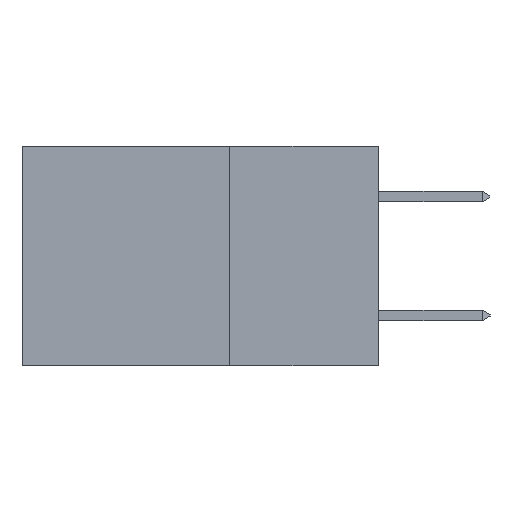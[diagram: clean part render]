
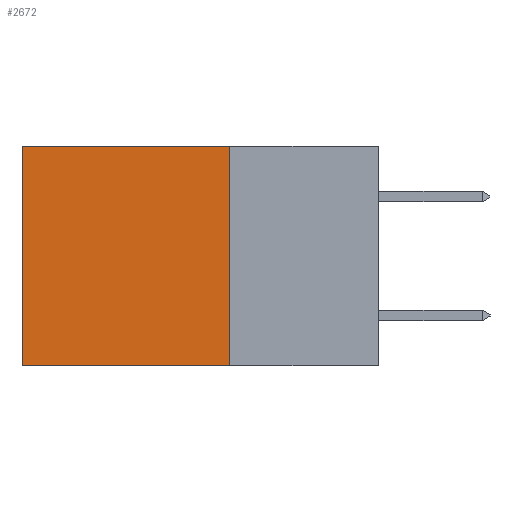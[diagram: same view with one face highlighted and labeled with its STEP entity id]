
A CAD part, left-side view. The second image highlights one B-rep face of the part: STEP entity #2672.
In plain terms, the highlighted planar face has unit normal (-1, 0, 0).
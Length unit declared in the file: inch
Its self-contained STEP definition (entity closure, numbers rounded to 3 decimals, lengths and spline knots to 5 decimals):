
#206 = AXIS2_PLACEMENT_3D ( 'NONE', #6173, #8094, #4147 ) ;
#280 = CARTESIAN_POINT ( 'NONE',  ( 0.2615, 0.25, -0.37 ) ) ;
#621 = EDGE_CURVE ( 'NONE', #991, #4308, #4250, .T. ) ;
#991 = VERTEX_POINT ( 'NONE', #280 ) ;
#1188 = DIRECTION ( 'NONE',  ( 0., 0., -1. ) ) ;
#1321 = CARTESIAN_POINT ( 'NONE',  ( 0.2615, 0.6, -0.37 ) ) ;
#1491 = EDGE_CURVE ( 'NONE', #3774, #991, #6326, .T. ) ;
#1506 = CARTESIAN_POINT ( 'NONE',  ( 0.2615, 0.25, -0.37 ) ) ;
#1646 = LINE ( 'NONE', #1321, #3534 ) ;
#2672 = ADVANCED_FACE ( 'NONE', ( #2991 ), #7448, .F. ) ;
#2991 = FACE_OUTER_BOUND ( 'NONE', #8503, .T. ) ;
#3029 = ORIENTED_EDGE ( 'NONE', *, *, #5022, .T. ) ;
#3534 = VECTOR ( 'NONE', #3707, 39.37008 ) ;
#3707 = DIRECTION ( 'NONE',  ( 0., 0., -1. ) ) ;
#3774 = VERTEX_POINT ( 'NONE', #5849 ) ;
#4147 = DIRECTION ( 'NONE',  ( 0., 0., -1. ) ) ;
#4250 = LINE ( 'NONE', #8840, #7572 ) ;
#4308 = VERTEX_POINT ( 'NONE', #5204 ) ;
#4875 = DIRECTION ( 'NONE',  ( 0., 1., 0. ) ) ;
#5022 = EDGE_CURVE ( 'NONE', #3774, #5112, #8647, .T. ) ;
#5112 = VERTEX_POINT ( 'NONE', #6967 ) ;
#5204 = CARTESIAN_POINT ( 'NONE',  ( 0.2615, 0.6, -0.37 ) ) ;
#5849 = CARTESIAN_POINT ( 'NONE',  ( 0.2615, 0.25, 0. ) ) ;
#6125 = VECTOR ( 'NONE', #1188, 39.37008 ) ;
#6173 = CARTESIAN_POINT ( 'NONE',  ( 0.2615, 0.25, -0.37 ) ) ;
#6222 = ORIENTED_EDGE ( 'NONE', *, *, #6470, .T. ) ;
#6326 = LINE ( 'NONE', #1506, #6125 ) ;
#6470 = EDGE_CURVE ( 'NONE', #5112, #4308, #1646, .T. ) ;
#6821 = ORIENTED_EDGE ( 'NONE', *, *, #621, .F. ) ;
#6967 = CARTESIAN_POINT ( 'NONE',  ( 0.2615, 0.6, 0. ) ) ;
#7337 = DIRECTION ( 'NONE',  ( 0., 1., 0. ) ) ;
#7448 = PLANE ( 'NONE',  #206 ) ;
#7572 = VECTOR ( 'NONE', #7337, 39.37008 ) ;
#8094 = DIRECTION ( 'NONE',  ( 1., 0., 0. ) ) ;
#8448 = VECTOR ( 'NONE', #4875, 39.37008 ) ;
#8503 = EDGE_LOOP ( 'NONE', ( #6222, #6821, #9101, #3029 ) ) ;
#8647 = LINE ( 'NONE', #8783, #8448 ) ;
#8783 = CARTESIAN_POINT ( 'NONE',  ( 0.2615, 0.25, 0. ) ) ;
#8840 = CARTESIAN_POINT ( 'NONE',  ( 0.2615, 0.25, -0.37 ) ) ;
#9101 = ORIENTED_EDGE ( 'NONE', *, *, #1491, .F. ) ;
